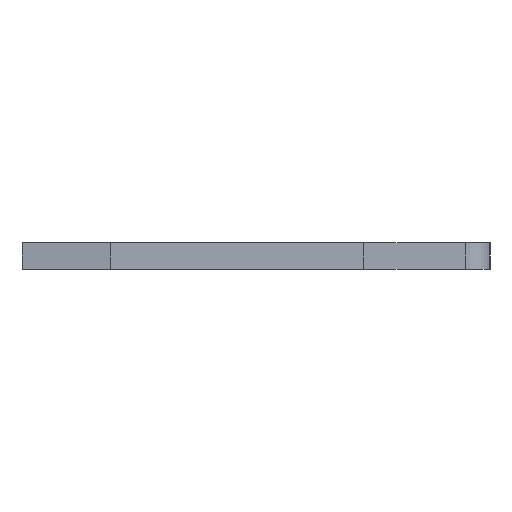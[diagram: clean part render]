
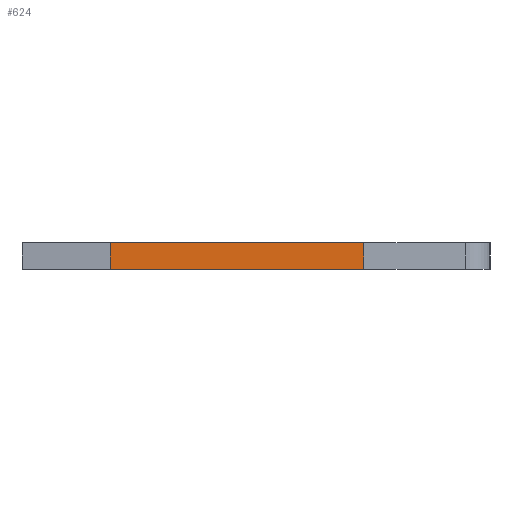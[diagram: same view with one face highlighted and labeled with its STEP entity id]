
A CAD part, left-side view. The second image highlights one B-rep face of the part: STEP entity #624.
In plain terms, the highlighted face is planar.
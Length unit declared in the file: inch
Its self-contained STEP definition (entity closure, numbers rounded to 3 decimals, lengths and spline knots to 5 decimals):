
#124 = DIRECTION ( 'NONE',  ( 0., 1., 0. ) ) ;
#209 = AXIS2_PLACEMENT_3D ( 'NONE', #1216, #268, #2009 ) ;
#268 = DIRECTION ( 'NONE',  ( 0., 0., 1. ) ) ;
#287 = CARTESIAN_POINT ( 'NONE',  ( -0.013, 0.146, -0.0575 ) ) ;
#296 = VERTEX_POINT ( 'NONE', #1959 ) ;
#343 = VECTOR ( 'NONE', #903, 39.37008 ) ;
#362 = CARTESIAN_POINT ( 'NONE',  ( -0.013, 0.146, -0.0575 ) ) ;
#481 = ORIENTED_EDGE ( 'NONE', *, *, #566, .T. ) ;
#553 = VERTEX_POINT ( 'NONE', #683 ) ;
#566 = EDGE_CURVE ( 'NONE', #1410, #553, #938, .T. ) ;
#590 = ORIENTED_EDGE ( 'NONE', *, *, #893, .F. ) ;
#624 = ADVANCED_FACE ( 'NONE', ( #1023 ), #1055, .F. ) ;
#683 = CARTESIAN_POINT ( 'NONE',  ( -0.013, -0.099, -0.0575 ) ) ;
#728 = CARTESIAN_POINT ( 'NONE',  ( 0.013, -0.099, -0.0575 ) ) ;
#760 = LINE ( 'NONE', #1658, #1698 ) ;
#796 = LINE ( 'NONE', #287, #1376 ) ;
#817 = ORIENTED_EDGE ( 'NONE', *, *, #971, .T. ) ;
#893 = EDGE_CURVE ( 'NONE', #1410, #296, #760, .T. ) ;
#903 = DIRECTION ( 'NONE',  ( -1., 0., 0. ) ) ;
#938 = LINE ( 'NONE', #728, #343 ) ;
#971 = EDGE_CURVE ( 'NONE', #553, #1397, #796, .T. ) ;
#993 = ORIENTED_EDGE ( 'NONE', *, *, #1233, .F. ) ;
#1014 = CARTESIAN_POINT ( 'NONE',  ( 0.013, -0.099, -0.0575 ) ) ;
#1023 = FACE_OUTER_BOUND ( 'NONE', #1525, .T. ) ;
#1055 = PLANE ( 'NONE',  #209 ) ;
#1216 = CARTESIAN_POINT ( 'NONE',  ( 0.013, 0.146, -0.0575 ) ) ;
#1233 = EDGE_CURVE ( 'NONE', #296, #1397, #1704, .T. ) ;
#1376 = VECTOR ( 'NONE', #2024, 39.37008 ) ;
#1397 = VERTEX_POINT ( 'NONE', #362 ) ;
#1410 = VERTEX_POINT ( 'NONE', #1014 ) ;
#1444 = CARTESIAN_POINT ( 'NONE',  ( 0.013, 0.146, -0.0575 ) ) ;
#1502 = VECTOR ( 'NONE', #1748, 39.37008 ) ;
#1525 = EDGE_LOOP ( 'NONE', ( #817, #993, #590, #481 ) ) ;
#1658 = CARTESIAN_POINT ( 'NONE',  ( 0.013, 0.146, -0.0575 ) ) ;
#1698 = VECTOR ( 'NONE', #124, 39.37008 ) ;
#1704 = LINE ( 'NONE', #1444, #1502 ) ;
#1748 = DIRECTION ( 'NONE',  ( -1., 0., 0. ) ) ;
#1959 = CARTESIAN_POINT ( 'NONE',  ( 0.013, 0.146, -0.0575 ) ) ;
#2009 = DIRECTION ( 'NONE',  ( 1., 0., 0. ) ) ;
#2024 = DIRECTION ( 'NONE',  ( 0., 1., 0. ) ) ;
